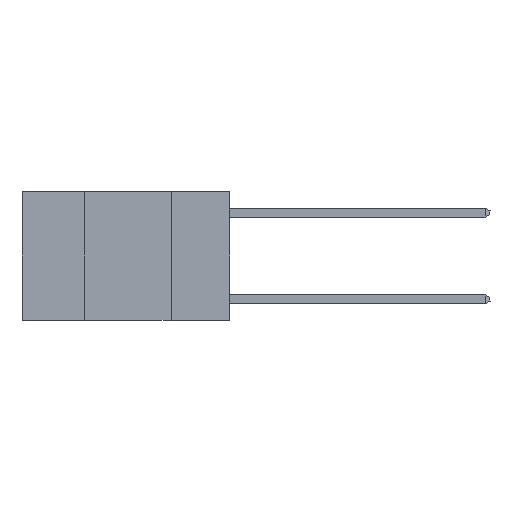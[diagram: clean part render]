
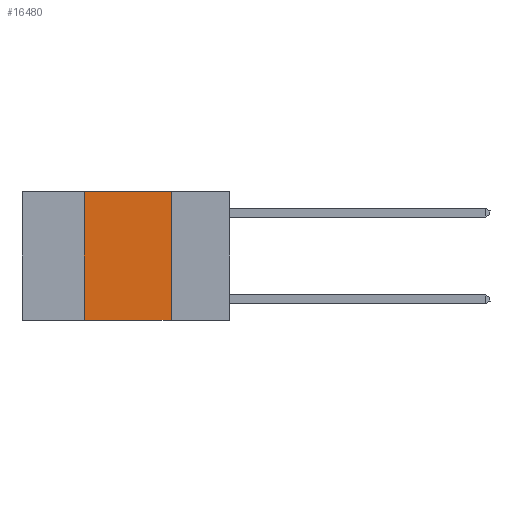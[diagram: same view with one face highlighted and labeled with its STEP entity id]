
A CAD part, left-side view. The second image highlights one B-rep face of the part: STEP entity #16480.
In plain terms, the highlighted planar face has unit normal (-1, 0, 0).
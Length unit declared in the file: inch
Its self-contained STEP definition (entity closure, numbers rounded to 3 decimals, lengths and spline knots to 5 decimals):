
#392 = VERTEX_POINT ( 'NONE', #12603 ) ;
#2375 = LINE ( 'NONE', #24773, #24785 ) ;
#4176 = DIRECTION ( 'NONE',  ( 0., 0., -1. ) ) ;
#4291 = DIRECTION ( 'NONE',  ( 0., -1., 0. ) ) ;
#4842 = VECTOR ( 'NONE', #4176, 39.37008 ) ;
#5022 = DIRECTION ( 'NONE',  ( 1., 0., 0. ) ) ;
#6560 = DIRECTION ( 'NONE',  ( 0., -1., 0. ) ) ;
#9099 = AXIS2_PLACEMENT_3D ( 'NONE', #11456, #5022, #20220 ) ;
#9168 = VERTEX_POINT ( 'NONE', #18777 ) ;
#9332 = ORIENTED_EDGE ( 'NONE', *, *, #23387, .T. ) ;
#9402 = CARTESIAN_POINT ( 'NONE',  ( 0., 0.42, -0.37 ) ) ;
#9738 = EDGE_LOOP ( 'NONE', ( #13060, #18864, #25958, #9332 ) ) ;
#10101 = EDGE_CURVE ( 'NONE', #392, #13207, #21259, .T. ) ;
#10608 = CARTESIAN_POINT ( 'NONE',  ( 0., 0.17, 0. ) ) ;
#11456 = CARTESIAN_POINT ( 'NONE',  ( 0., 0.6, 0. ) ) ;
#12603 = CARTESIAN_POINT ( 'NONE',  ( 0., 0.42, 0. ) ) ;
#12853 = EDGE_CURVE ( 'NONE', #13207, #9168, #20801, .T. ) ;
#13060 = ORIENTED_EDGE ( 'NONE', *, *, #12853, .F. ) ;
#13207 = VERTEX_POINT ( 'NONE', #20474 ) ;
#15106 = CARTESIAN_POINT ( 'NONE',  ( 0., 0.6, 0. ) ) ;
#16480 = ADVANCED_FACE ( 'NONE', ( #23734 ), #18023, .F. ) ;
#17422 = CARTESIAN_POINT ( 'NONE',  ( 0., 0.6, -0.37 ) ) ;
#17570 = LINE ( 'NONE', #17422, #22645 ) ;
#18023 = PLANE ( 'NONE',  #9099 ) ;
#18777 = CARTESIAN_POINT ( 'NONE',  ( 0., 0.17, -0.37 ) ) ;
#18864 = ORIENTED_EDGE ( 'NONE', *, *, #10101, .F. ) ;
#20220 = DIRECTION ( 'NONE',  ( 0., 0., -1. ) ) ;
#20474 = CARTESIAN_POINT ( 'NONE',  ( 0., 0.17, 0. ) ) ;
#20801 = LINE ( 'NONE', #10608, #4842 ) ;
#21259 = LINE ( 'NONE', #15106, #26322 ) ;
#21907 = EDGE_CURVE ( 'NONE', #23577, #392, #2375, .T. ) ;
#22645 = VECTOR ( 'NONE', #6560, 39.37008 ) ;
#23387 = EDGE_CURVE ( 'NONE', #23577, #9168, #17570, .T. ) ;
#23577 = VERTEX_POINT ( 'NONE', #9402 ) ;
#23734 = FACE_OUTER_BOUND ( 'NONE', #9738, .T. ) ;
#24773 = CARTESIAN_POINT ( 'NONE',  ( 0., 0.42, 0. ) ) ;
#24785 = VECTOR ( 'NONE', #26903, 39.37008 ) ;
#25958 = ORIENTED_EDGE ( 'NONE', *, *, #21907, .F. ) ;
#26322 = VECTOR ( 'NONE', #4291, 39.37008 ) ;
#26903 = DIRECTION ( 'NONE',  ( 0., 0., 1. ) ) ;
